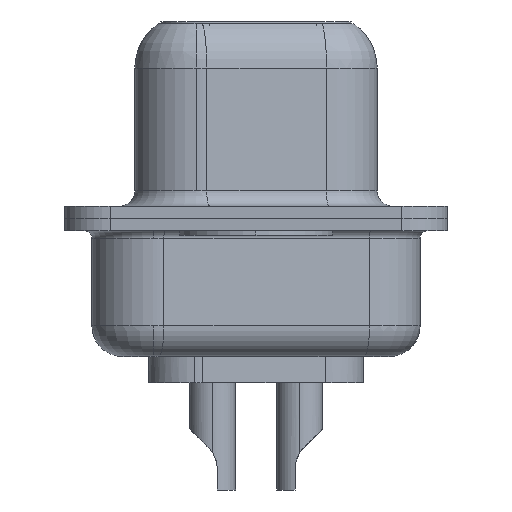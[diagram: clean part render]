
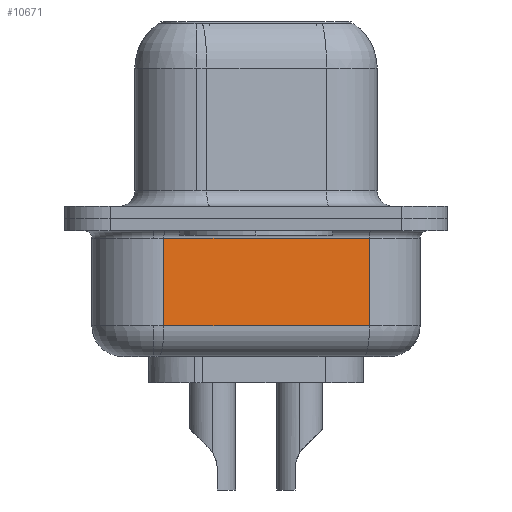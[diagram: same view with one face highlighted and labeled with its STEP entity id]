
A CAD part, left-side view. The second image highlights one B-rep face of the part: STEP entity #10671.
In plain terms, the highlighted planar face has unit normal (-0.985, -0.174, 0).
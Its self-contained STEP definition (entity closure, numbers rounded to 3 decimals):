
#994 = EDGE_CURVE ( 'NONE', #7285, #14138, #3967, .T. ) ;
#1263 = EDGE_LOOP ( 'NONE', ( #7361, #6954, #3775, #3220 ) ) ;
#1374 = LINE ( 'NONE', #3826, #10280 ) ;
#2329 = PLANE ( 'NONE',  #15658 ) ;
#2371 = VECTOR ( 'NONE', #15758, 1000. ) ;
#2658 = CARTESIAN_POINT ( 'NONE',  ( 2.88, 3.003, -0.65 ) ) ;
#3220 = ORIENTED_EDGE ( 'NONE', *, *, #994, .T. ) ;
#3742 = CARTESIAN_POINT ( 'NONE',  ( 4.062, -3.697, -0.65 ) ) ;
#3775 = ORIENTED_EDGE ( 'NONE', *, *, #4050, .T. ) ;
#3826 = CARTESIAN_POINT ( 'NONE',  ( 2.88, 3.003, -3.5 ) ) ;
#3967 = LINE ( 'NONE', #2658, #7594 ) ;
#4050 = EDGE_CURVE ( 'NONE', #7244, #7285, #5774, .T. ) ;
#5085 = CARTESIAN_POINT ( 'NONE',  ( 2.88, 3.003, -4.5 ) ) ;
#5774 = LINE ( 'NONE', #10782, #2371 ) ;
#5928 = CARTESIAN_POINT ( 'NONE',  ( 2.88, 3.003, -3.5 ) ) ;
#6240 = DIRECTION ( 'NONE',  ( -0.174, 0.985, 0. ) ) ;
#6591 = EDGE_CURVE ( 'NONE', #11758, #14138, #8155, .T. ) ;
#6954 = ORIENTED_EDGE ( 'NONE', *, *, #7192, .T. ) ;
#7192 = EDGE_CURVE ( 'NONE', #11758, #7244, #1374, .T. ) ;
#7244 = VERTEX_POINT ( 'NONE', #10047 ) ;
#7285 = VERTEX_POINT ( 'NONE', #3742 ) ;
#7361 = ORIENTED_EDGE ( 'NONE', *, *, #6591, .F. ) ;
#7594 = VECTOR ( 'NONE', #12726, 1000. ) ;
#8155 = LINE ( 'NONE', #15687, #10813 ) ;
#10047 = CARTESIAN_POINT ( 'NONE',  ( 4.062, -3.697, -3.5 ) ) ;
#10089 = DIRECTION ( 'NONE',  ( 0.985, 0.174, 0. ) ) ;
#10280 = VECTOR ( 'NONE', #13819, 1000. ) ;
#10671 = ADVANCED_FACE ( 'NONE', ( #11169 ), #2329, .F. ) ;
#10782 = CARTESIAN_POINT ( 'NONE',  ( 4.062, -3.697, -4.5 ) ) ;
#10813 = VECTOR ( 'NONE', #14551, 1000. ) ;
#11169 = FACE_OUTER_BOUND ( 'NONE', #1263, .T. ) ;
#11758 = VERTEX_POINT ( 'NONE', #5928 ) ;
#12726 = DIRECTION ( 'NONE',  ( -0.174, 0.985, 0. ) ) ;
#13004 = CARTESIAN_POINT ( 'NONE',  ( 2.88, 3.003, -0.65 ) ) ;
#13819 = DIRECTION ( 'NONE',  ( 0.174, -0.985, 0. ) ) ;
#14138 = VERTEX_POINT ( 'NONE', #13004 ) ;
#14551 = DIRECTION ( 'NONE',  ( 0., 0., 1. ) ) ;
#15658 = AXIS2_PLACEMENT_3D ( 'NONE', #5085, #10089, #6240 ) ;
#15687 = CARTESIAN_POINT ( 'NONE',  ( 2.88, 3.003, -4.5 ) ) ;
#15758 = DIRECTION ( 'NONE',  ( 0., 0., 1. ) ) ;
